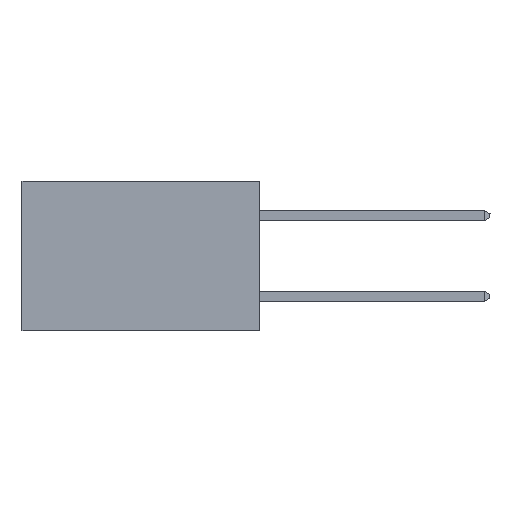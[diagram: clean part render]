
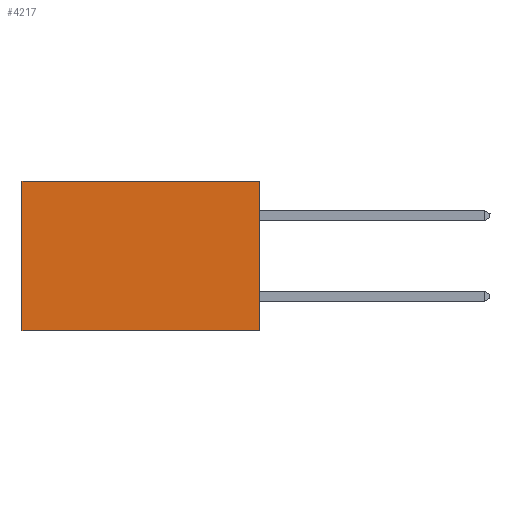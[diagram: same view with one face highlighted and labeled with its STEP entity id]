
A CAD part, left-side view. The second image highlights one B-rep face of the part: STEP entity #4217.
In plain terms, the highlighted planar face has unit normal (-1, 0, 0).
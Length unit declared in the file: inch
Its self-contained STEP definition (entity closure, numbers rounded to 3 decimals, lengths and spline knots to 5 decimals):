
#19 = CARTESIAN_POINT ( 'NONE',  ( 0.277, 0., -0.37 ) ) ;
#537 = ORIENTED_EDGE ( 'NONE', *, *, #6809, .F. ) ;
#548 = VERTEX_POINT ( 'NONE', #11708 ) ;
#594 = AXIS2_PLACEMENT_3D ( 'NONE', #10725, #10555, #10538 ) ;
#1122 = ORIENTED_EDGE ( 'NONE', *, *, #7733, .T. ) ;
#1124 = DIRECTION ( 'NONE',  ( 0., 0., -1. ) ) ;
#1545 = EDGE_CURVE ( 'NONE', #5617, #9196, #7254, .T. ) ;
#1967 = LINE ( 'NONE', #5303, #11293 ) ;
#2104 = LINE ( 'NONE', #4421, #9333 ) ;
#2110 = ORIENTED_EDGE ( 'NONE', *, *, #1545, .F. ) ;
#3020 = DIRECTION ( 'NONE',  ( 0., 1., 0. ) ) ;
#4217 = ADVANCED_FACE ( 'NONE', ( #8340 ), #10574, .F. ) ;
#4421 = CARTESIAN_POINT ( 'NONE',  ( 0.277, 0., 0. ) ) ;
#4632 = ORIENTED_EDGE ( 'NONE', *, *, #5641, .T. ) ;
#5303 = CARTESIAN_POINT ( 'NONE',  ( 0.277, 0., -0.37 ) ) ;
#5515 = CARTESIAN_POINT ( 'NONE',  ( 0.277, 0., -0.37 ) ) ;
#5575 = LINE ( 'NONE', #6316, #7743 ) ;
#5617 = VERTEX_POINT ( 'NONE', #19 ) ;
#5641 = EDGE_CURVE ( 'NONE', #548, #9196, #5575, .T. ) ;
#6162 = DIRECTION ( 'NONE',  ( 0., 0., -1. ) ) ;
#6316 = CARTESIAN_POINT ( 'NONE',  ( 0.277, 0.59, -0.37 ) ) ;
#6547 = DIRECTION ( 'NONE',  ( 0., 1., 0. ) ) ;
#6809 = EDGE_CURVE ( 'NONE', #10774, #5617, #1967, .T. ) ;
#7254 = LINE ( 'NONE', #5515, #9367 ) ;
#7733 = EDGE_CURVE ( 'NONE', #10774, #548, #2104, .T. ) ;
#7743 = VECTOR ( 'NONE', #1124, 39.37008 ) ;
#8340 = FACE_OUTER_BOUND ( 'NONE', #11042, .T. ) ;
#9196 = VERTEX_POINT ( 'NONE', #10068 ) ;
#9333 = VECTOR ( 'NONE', #3020, 39.37008 ) ;
#9367 = VECTOR ( 'NONE', #6547, 39.37008 ) ;
#10068 = CARTESIAN_POINT ( 'NONE',  ( 0.277, 0.59, -0.37 ) ) ;
#10538 = DIRECTION ( 'NONE',  ( 0., 0., -1. ) ) ;
#10555 = DIRECTION ( 'NONE',  ( 1., 0., 0. ) ) ;
#10574 = PLANE ( 'NONE',  #594 ) ;
#10725 = CARTESIAN_POINT ( 'NONE',  ( 0.277, 0., -0.37 ) ) ;
#10774 = VERTEX_POINT ( 'NONE', #10794 ) ;
#10794 = CARTESIAN_POINT ( 'NONE',  ( 0.277, 0., 0. ) ) ;
#11042 = EDGE_LOOP ( 'NONE', ( #4632, #2110, #537, #1122 ) ) ;
#11293 = VECTOR ( 'NONE', #6162, 39.37008 ) ;
#11708 = CARTESIAN_POINT ( 'NONE',  ( 0.277, 0.59, 0. ) ) ;
